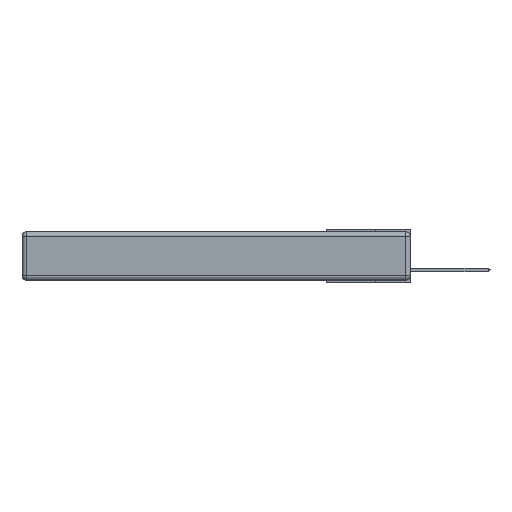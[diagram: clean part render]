
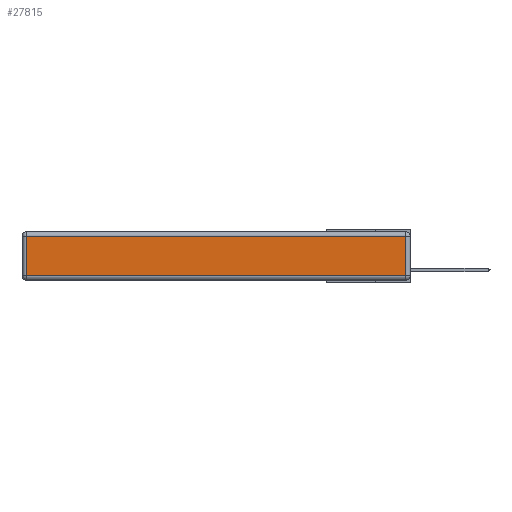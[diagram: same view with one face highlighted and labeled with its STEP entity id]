
A CAD part, left-side view. The second image highlights one B-rep face of the part: STEP entity #27815.
In plain terms, the highlighted planar face has unit normal (-1, 0, 0).
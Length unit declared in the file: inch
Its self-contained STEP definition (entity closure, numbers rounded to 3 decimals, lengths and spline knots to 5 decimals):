
#533 = DIRECTION ( 'NONE',  ( 0., 0., 1. ) ) ;
#3724 = VERTEX_POINT ( 'NONE', #15359 ) ;
#4165 = DIRECTION ( 'NONE',  ( 0., -1., 0. ) ) ;
#6448 = VECTOR ( 'NONE', #13827, 39.37008 ) ;
#6988 = DIRECTION ( 'NONE',  ( 0., 1., 0. ) ) ;
#7795 = LINE ( 'NONE', #11496, #26434 ) ;
#8016 = AXIS2_PLACEMENT_3D ( 'NONE', #14139, #19748, #533 ) ;
#10379 = ORIENTED_EDGE ( 'NONE', *, *, #11028, .T. ) ;
#10833 = VECTOR ( 'NONE', #6988, 39.37008 ) ;
#11028 = EDGE_CURVE ( 'NONE', #25591, #16177, #19065, .T. ) ;
#11468 = ORIENTED_EDGE ( 'NONE', *, *, #15409, .T. ) ;
#11496 = CARTESIAN_POINT ( 'NONE',  ( 0., 0., -0.313 ) ) ;
#13023 = CARTESIAN_POINT ( 'NONE',  ( 0., 0.03, -0.03 ) ) ;
#13827 = DIRECTION ( 'NONE',  ( 0., 0., -1. ) ) ;
#14139 = CARTESIAN_POINT ( 'NONE',  ( 0., 0., -0.343 ) ) ;
#15359 = CARTESIAN_POINT ( 'NONE',  ( 0., 2.72, -0.03 ) ) ;
#15409 = EDGE_CURVE ( 'NONE', #17687, #25591, #7795, .T. ) ;
#16177 = VERTEX_POINT ( 'NONE', #13023 ) ;
#16348 = CARTESIAN_POINT ( 'NONE',  ( 0., 2.75, -0.03 ) ) ;
#16470 = VECTOR ( 'NONE', #20263, 39.37008 ) ;
#17687 = VERTEX_POINT ( 'NONE', #20380 ) ;
#18508 = CARTESIAN_POINT ( 'NONE',  ( 0., 2.72, -0.343 ) ) ;
#19065 = LINE ( 'NONE', #19865, #16470 ) ;
#19114 = LINE ( 'NONE', #18508, #6448 ) ;
#19429 = LINE ( 'NONE', #16348, #10833 ) ;
#19664 = EDGE_CURVE ( 'NONE', #3724, #17687, #19114, .T. ) ;
#19748 = DIRECTION ( 'NONE',  ( -1., 0., 0. ) ) ;
#19865 = CARTESIAN_POINT ( 'NONE',  ( 0., 0.03, -0.343 ) ) ;
#20263 = DIRECTION ( 'NONE',  ( 0., 0., 1. ) ) ;
#20380 = CARTESIAN_POINT ( 'NONE',  ( 0., 2.72, -0.313 ) ) ;
#21093 = EDGE_CURVE ( 'NONE', #16177, #3724, #19429, .T. ) ;
#21144 = CARTESIAN_POINT ( 'NONE',  ( 0., 0.03, -0.313 ) ) ;
#22361 = ORIENTED_EDGE ( 'NONE', *, *, #19664, .T. ) ;
#25591 = VERTEX_POINT ( 'NONE', #21144 ) ;
#26014 = ORIENTED_EDGE ( 'NONE', *, *, #21093, .T. ) ;
#26434 = VECTOR ( 'NONE', #4165, 39.37008 ) ;
#27358 = FACE_OUTER_BOUND ( 'NONE', #29141, .T. ) ;
#27815 = ADVANCED_FACE ( 'NONE', ( #27358 ), #28403, .T. ) ;
#28403 = PLANE ( 'NONE',  #8016 ) ;
#29141 = EDGE_LOOP ( 'NONE', ( #11468, #10379, #26014, #22361 ) ) ;
